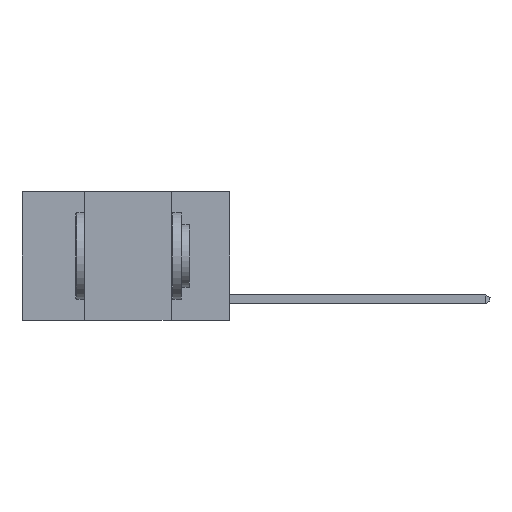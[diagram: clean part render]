
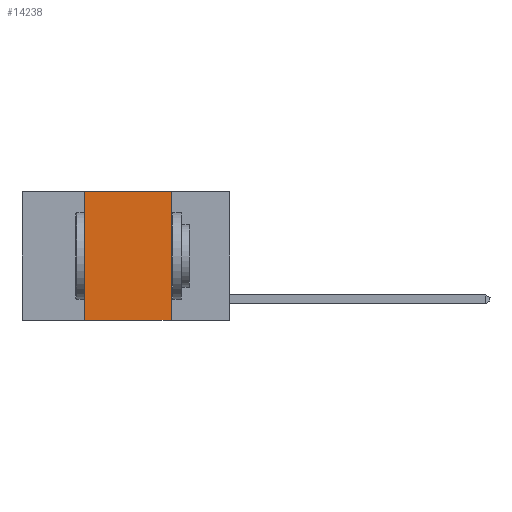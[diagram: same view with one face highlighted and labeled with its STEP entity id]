
A CAD part, left-side view. The second image highlights one B-rep face of the part: STEP entity #14238.
In plain terms, the highlighted planar face has unit normal (-1, 0, 0).
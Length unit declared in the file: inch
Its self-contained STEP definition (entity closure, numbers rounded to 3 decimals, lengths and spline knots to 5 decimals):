
#530 = LINE ( 'NONE', #2715, #7641 ) ;
#1004 = EDGE_CURVE ( 'NONE', #16615, #8209, #530, .T. ) ;
#1126 = DIRECTION ( 'NONE',  ( 0., 0., -1. ) ) ;
#1569 = PLANE ( 'NONE',  #2728 ) ;
#1713 = LINE ( 'NONE', #9059, #3741 ) ;
#2489 = EDGE_LOOP ( 'NONE', ( #23002, #23703, #16419, #19583 ) ) ;
#2715 = CARTESIAN_POINT ( 'NONE',  ( 0., 0.6, -0.37 ) ) ;
#2728 = AXIS2_PLACEMENT_3D ( 'NONE', #15722, #4748, #1126 ) ;
#3379 = VERTEX_POINT ( 'NONE', #10128 ) ;
#3741 = VECTOR ( 'NONE', #15967, 39.37008 ) ;
#4423 = CARTESIAN_POINT ( 'NONE',  ( 0., 0.17, -0.37 ) ) ;
#4748 = DIRECTION ( 'NONE',  ( 1., 0., 0. ) ) ;
#5435 = CARTESIAN_POINT ( 'NONE',  ( 0., 0.6, 0. ) ) ;
#6818 = VECTOR ( 'NONE', #18500, 39.37008 ) ;
#7641 = VECTOR ( 'NONE', #15490, 39.37008 ) ;
#8209 = VERTEX_POINT ( 'NONE', #4423 ) ;
#8977 = EDGE_CURVE ( 'NONE', #16615, #19687, #1713, .T. ) ;
#9059 = CARTESIAN_POINT ( 'NONE',  ( 0., 0.42, 0. ) ) ;
#9522 = EDGE_CURVE ( 'NONE', #19687, #3379, #16772, .T. ) ;
#10128 = CARTESIAN_POINT ( 'NONE',  ( 0., 0.17, 0. ) ) ;
#14238 = ADVANCED_FACE ( 'NONE', ( #15852 ), #1569, .F. ) ;
#14669 = DIRECTION ( 'NONE',  ( 0., 0., -1. ) ) ;
#15490 = DIRECTION ( 'NONE',  ( 0., -1., 0. ) ) ;
#15722 = CARTESIAN_POINT ( 'NONE',  ( 0., 0.6, 0. ) ) ;
#15852 = FACE_OUTER_BOUND ( 'NONE', #2489, .T. ) ;
#15967 = DIRECTION ( 'NONE',  ( 0., 0., 1. ) ) ;
#16419 = ORIENTED_EDGE ( 'NONE', *, *, #8977, .F. ) ;
#16615 = VERTEX_POINT ( 'NONE', #20952 ) ;
#16772 = LINE ( 'NONE', #5435, #6818 ) ;
#17136 = VECTOR ( 'NONE', #14669, 39.37008 ) ;
#17641 = CARTESIAN_POINT ( 'NONE',  ( 0., 0.42, 0. ) ) ;
#18500 = DIRECTION ( 'NONE',  ( 0., -1., 0. ) ) ;
#19583 = ORIENTED_EDGE ( 'NONE', *, *, #1004, .T. ) ;
#19687 = VERTEX_POINT ( 'NONE', #17641 ) ;
#19889 = CARTESIAN_POINT ( 'NONE',  ( 0., 0.17, 0. ) ) ;
#20229 = EDGE_CURVE ( 'NONE', #3379, #8209, #22093, .T. ) ;
#20952 = CARTESIAN_POINT ( 'NONE',  ( 0., 0.42, -0.37 ) ) ;
#22093 = LINE ( 'NONE', #19889, #17136 ) ;
#23002 = ORIENTED_EDGE ( 'NONE', *, *, #20229, .F. ) ;
#23703 = ORIENTED_EDGE ( 'NONE', *, *, #9522, .F. ) ;
